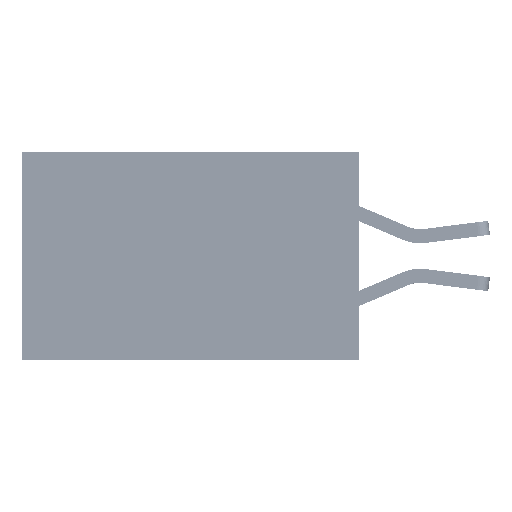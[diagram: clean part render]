
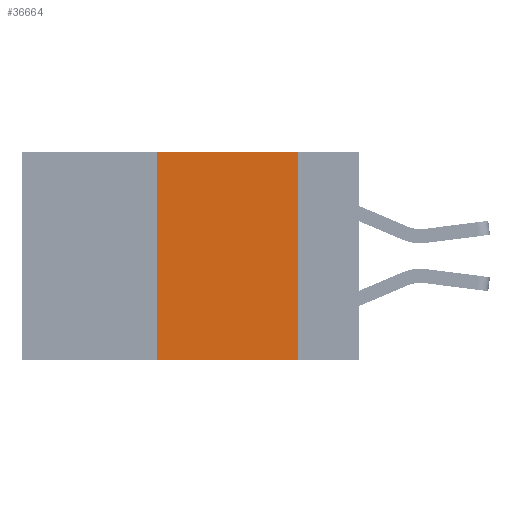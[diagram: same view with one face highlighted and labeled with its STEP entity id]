
A CAD part, left-side view. The second image highlights one B-rep face of the part: STEP entity #36664.
In plain terms, the highlighted planar face has unit normal (-1, 0, 0).
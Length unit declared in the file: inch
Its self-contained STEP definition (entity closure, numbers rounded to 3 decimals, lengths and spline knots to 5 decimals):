
#540 = VECTOR ( 'NONE', #6328, 39.37008 ) ;
#997 = PLANE ( 'NONE',  #24490 ) ;
#2706 = VERTEX_POINT ( 'NONE', #41824 ) ;
#2751 = CARTESIAN_POINT ( 'NONE',  ( 0., 0.36, 0. ) ) ;
#4938 = CARTESIAN_POINT ( 'NONE',  ( 0., 0.6, 0. ) ) ;
#5618 = EDGE_LOOP ( 'NONE', ( #17839, #12469, #12868, #9194 ) ) ;
#6328 = DIRECTION ( 'NONE',  ( 0., -1., 0. ) ) ;
#6485 = VECTOR ( 'NONE', #33719, 39.37008 ) ;
#6603 = CARTESIAN_POINT ( 'NONE',  ( 0., 0.36, 0. ) ) ;
#7575 = VECTOR ( 'NONE', #14088, 39.37008 ) ;
#7606 = DIRECTION ( 'NONE',  ( 0., -1., 0. ) ) ;
#9194 = ORIENTED_EDGE ( 'NONE', *, *, #26136, .T. ) ;
#9681 = LINE ( 'NONE', #37037, #540 ) ;
#10990 = CARTESIAN_POINT ( 'NONE',  ( 0., 0.11, 0. ) ) ;
#12364 = CARTESIAN_POINT ( 'NONE',  ( 0., 0.11, -0.37 ) ) ;
#12469 = ORIENTED_EDGE ( 'NONE', *, *, #15954, .F. ) ;
#12868 = ORIENTED_EDGE ( 'NONE', *, *, #25911, .F. ) ;
#13887 = LINE ( 'NONE', #19349, #7575 ) ;
#14088 = DIRECTION ( 'NONE',  ( 0., 0., -1. ) ) ;
#15885 = VERTEX_POINT ( 'NONE', #10990 ) ;
#15954 = EDGE_CURVE ( 'NONE', #27179, #15885, #17941, .T. ) ;
#16901 = EDGE_CURVE ( 'NONE', #15885, #18367, #13887, .T. ) ;
#17839 = ORIENTED_EDGE ( 'NONE', *, *, #16901, .F. ) ;
#17941 = LINE ( 'NONE', #4938, #22091 ) ;
#18367 = VERTEX_POINT ( 'NONE', #12364 ) ;
#19349 = CARTESIAN_POINT ( 'NONE',  ( 0., 0.11, 0. ) ) ;
#20953 = DIRECTION ( 'NONE',  ( 1., 0., 0. ) ) ;
#22091 = VECTOR ( 'NONE', #7606, 39.37008 ) ;
#24490 = AXIS2_PLACEMENT_3D ( 'NONE', #41796, #20953, #41346 ) ;
#25911 = EDGE_CURVE ( 'NONE', #2706, #27179, #37092, .T. ) ;
#26136 = EDGE_CURVE ( 'NONE', #2706, #18367, #9681, .T. ) ;
#27179 = VERTEX_POINT ( 'NONE', #2751 ) ;
#31030 = FACE_OUTER_BOUND ( 'NONE', #5618, .T. ) ;
#33719 = DIRECTION ( 'NONE',  ( 0., 0., 1. ) ) ;
#36664 = ADVANCED_FACE ( 'NONE', ( #31030 ), #997, .F. ) ;
#37037 = CARTESIAN_POINT ( 'NONE',  ( 0., 0.6, -0.37 ) ) ;
#37092 = LINE ( 'NONE', #6603, #6485 ) ;
#41346 = DIRECTION ( 'NONE',  ( 0., 0., -1. ) ) ;
#41796 = CARTESIAN_POINT ( 'NONE',  ( 0., 0.6, 0. ) ) ;
#41824 = CARTESIAN_POINT ( 'NONE',  ( 0., 0.36, -0.37 ) ) ;
